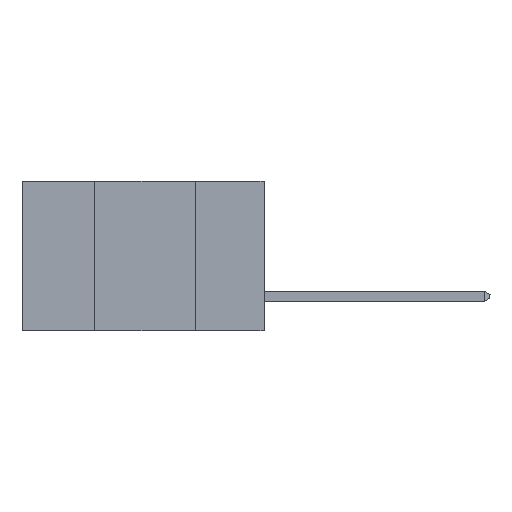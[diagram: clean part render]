
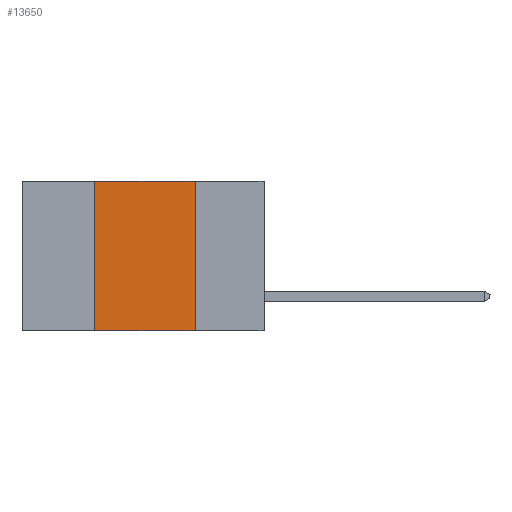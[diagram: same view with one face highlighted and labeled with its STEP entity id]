
A CAD part, left-side view. The second image highlights one B-rep face of the part: STEP entity #13650.
In plain terms, the highlighted planar face has unit normal (-1, 0, 0).
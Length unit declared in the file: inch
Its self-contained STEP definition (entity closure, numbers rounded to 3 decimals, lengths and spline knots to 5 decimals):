
#7 = DIRECTION ( 'NONE',  ( 0., 0., -1. ) ) ;
#179 = LINE ( 'NONE', #10430, #5255 ) ;
#524 = DIRECTION ( 'NONE',  ( 0., 0., -1. ) ) ;
#668 = EDGE_CURVE ( 'NONE', #6873, #15981, #7628, .T. ) ;
#764 = PLANE ( 'NONE',  #8048 ) ;
#1012 = VECTOR ( 'NONE', #7, 39.37008 ) ;
#1276 = CARTESIAN_POINT ( 'NONE',  ( 0., 0.42, 0. ) ) ;
#2078 = VECTOR ( 'NONE', #12866, 39.37008 ) ;
#2295 = CARTESIAN_POINT ( 'NONE',  ( 0., 0.6, 0. ) ) ;
#3086 = FACE_OUTER_BOUND ( 'NONE', #8926, .T. ) ;
#3567 = ORIENTED_EDGE ( 'NONE', *, *, #668, .T. ) ;
#4756 = EDGE_CURVE ( 'NONE', #15062, #15170, #6845, .T. ) ;
#5255 = VECTOR ( 'NONE', #6914, 39.37008 ) ;
#6845 = LINE ( 'NONE', #2295, #6921 ) ;
#6873 = VERTEX_POINT ( 'NONE', #16329 ) ;
#6914 = DIRECTION ( 'NONE',  ( 0., 0., 1. ) ) ;
#6921 = VECTOR ( 'NONE', #9932, 39.37008 ) ;
#7297 = ORIENTED_EDGE ( 'NONE', *, *, #4756, .F. ) ;
#7628 = LINE ( 'NONE', #9744, #2078 ) ;
#7686 = CARTESIAN_POINT ( 'NONE',  ( 0., 0.17, -0.37 ) ) ;
#8026 = CARTESIAN_POINT ( 'NONE',  ( 0., 0.17, 0. ) ) ;
#8048 = AXIS2_PLACEMENT_3D ( 'NONE', #13533, #11128, #524 ) ;
#8926 = EDGE_LOOP ( 'NONE', ( #12895, #7297, #14188, #3567 ) ) ;
#9744 = CARTESIAN_POINT ( 'NONE',  ( 0., 0.6, -0.37 ) ) ;
#9932 = DIRECTION ( 'NONE',  ( 0., -1., 0. ) ) ;
#10430 = CARTESIAN_POINT ( 'NONE',  ( 0., 0.42, -0.37 ) ) ;
#11128 = DIRECTION ( 'NONE',  ( 1., 0., 0. ) ) ;
#11648 = LINE ( 'NONE', #7686, #1012 ) ;
#12866 = DIRECTION ( 'NONE',  ( 0., -1., 0. ) ) ;
#12895 = ORIENTED_EDGE ( 'NONE', *, *, #12921, .F. ) ;
#12921 = EDGE_CURVE ( 'NONE', #15170, #15981, #11648, .T. ) ;
#13533 = CARTESIAN_POINT ( 'NONE',  ( 0., 0.6, 0. ) ) ;
#13650 = ADVANCED_FACE ( 'NONE', ( #3086 ), #764, .F. ) ;
#14188 = ORIENTED_EDGE ( 'NONE', *, *, #15174, .F. ) ;
#15062 = VERTEX_POINT ( 'NONE', #1276 ) ;
#15170 = VERTEX_POINT ( 'NONE', #8026 ) ;
#15174 = EDGE_CURVE ( 'NONE', #6873, #15062, #179, .T. ) ;
#15981 = VERTEX_POINT ( 'NONE', #16395 ) ;
#16329 = CARTESIAN_POINT ( 'NONE',  ( 0., 0.42, -0.37 ) ) ;
#16395 = CARTESIAN_POINT ( 'NONE',  ( 0., 0.17, -0.37 ) ) ;
